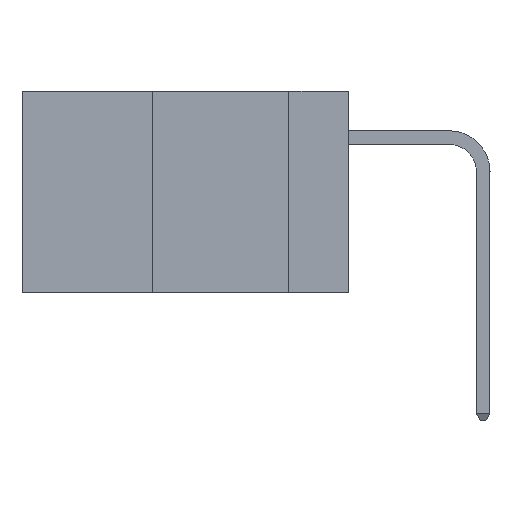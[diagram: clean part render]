
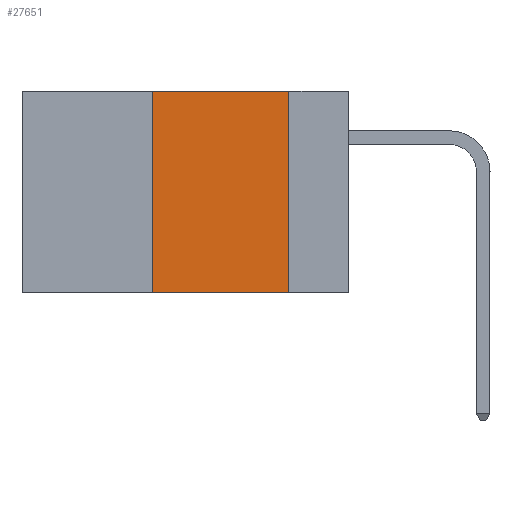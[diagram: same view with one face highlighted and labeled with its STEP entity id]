
A CAD part, left-side view. The second image highlights one B-rep face of the part: STEP entity #27651.
In plain terms, the highlighted planar face has unit normal (-1, 0, 0).
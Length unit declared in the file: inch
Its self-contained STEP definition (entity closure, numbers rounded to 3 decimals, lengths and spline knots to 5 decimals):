
#1659 = LINE ( 'NONE', #21486, #26955 ) ;
#3330 = VERTEX_POINT ( 'NONE', #13692 ) ;
#4814 = VECTOR ( 'NONE', #8663, 39.37008 ) ;
#4873 = DIRECTION ( 'NONE',  ( 1., 0., 0. ) ) ;
#6018 = DIRECTION ( 'NONE',  ( 0., -1., 0. ) ) ;
#6024 = ORIENTED_EDGE ( 'NONE', *, *, #10320, .F. ) ;
#6752 = CARTESIAN_POINT ( 'NONE',  ( 0., 0.36, 0. ) ) ;
#6862 = CARTESIAN_POINT ( 'NONE',  ( 0., 0.11, 0. ) ) ;
#8663 = DIRECTION ( 'NONE',  ( 0., -1., 0. ) ) ;
#10076 = ORIENTED_EDGE ( 'NONE', *, *, #25862, .T. ) ;
#10320 = EDGE_CURVE ( 'NONE', #30673, #31253, #18427, .T. ) ;
#11053 = VECTOR ( 'NONE', #22019, 39.37008 ) ;
#12849 = EDGE_LOOP ( 'NONE', ( #15971, #6024, #23523, #10076 ) ) ;
#13692 = CARTESIAN_POINT ( 'NONE',  ( 0., 0.36, -0.37 ) ) ;
#14155 = CARTESIAN_POINT ( 'NONE',  ( 0., 0.36, 0. ) ) ;
#15971 = ORIENTED_EDGE ( 'NONE', *, *, #30651, .F. ) ;
#16611 = DIRECTION ( 'NONE',  ( 0., 0., -1. ) ) ;
#17881 = LINE ( 'NONE', #6752, #11053 ) ;
#18427 = LINE ( 'NONE', #23815, #4814 ) ;
#19002 = FACE_OUTER_BOUND ( 'NONE', #12849, .T. ) ;
#20141 = CARTESIAN_POINT ( 'NONE',  ( 0., 0.6, 0. ) ) ;
#21486 = CARTESIAN_POINT ( 'NONE',  ( 0., 0.11, 0. ) ) ;
#22019 = DIRECTION ( 'NONE',  ( 0., 0., 1. ) ) ;
#22692 = DIRECTION ( 'NONE',  ( 0., 0., -1. ) ) ;
#23010 = AXIS2_PLACEMENT_3D ( 'NONE', #20141, #4873, #22692 ) ;
#23523 = ORIENTED_EDGE ( 'NONE', *, *, #27495, .F. ) ;
#23780 = CARTESIAN_POINT ( 'NONE',  ( 0., 0.6, -0.37 ) ) ;
#23815 = CARTESIAN_POINT ( 'NONE',  ( 0., 0.6, 0. ) ) ;
#25349 = VECTOR ( 'NONE', #6018, 39.37008 ) ;
#25862 = EDGE_CURVE ( 'NONE', #3330, #30615, #32433, .T. ) ;
#26326 = CARTESIAN_POINT ( 'NONE',  ( 0., 0.11, -0.37 ) ) ;
#26955 = VECTOR ( 'NONE', #16611, 39.37008 ) ;
#27495 = EDGE_CURVE ( 'NONE', #3330, #30673, #17881, .T. ) ;
#27651 = ADVANCED_FACE ( 'NONE', ( #19002 ), #29829, .F. ) ;
#29829 = PLANE ( 'NONE',  #23010 ) ;
#30615 = VERTEX_POINT ( 'NONE', #26326 ) ;
#30651 = EDGE_CURVE ( 'NONE', #31253, #30615, #1659, .T. ) ;
#30673 = VERTEX_POINT ( 'NONE', #14155 ) ;
#31253 = VERTEX_POINT ( 'NONE', #6862 ) ;
#32433 = LINE ( 'NONE', #23780, #25349 ) ;
